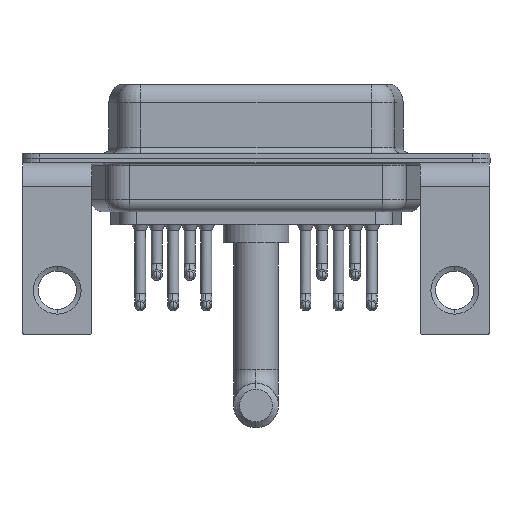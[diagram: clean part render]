
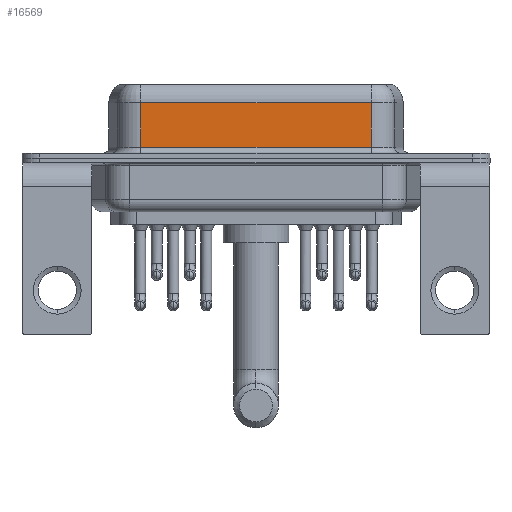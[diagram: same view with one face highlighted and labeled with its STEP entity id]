
A CAD part, front view. The second image highlights one B-rep face of the part: STEP entity #16569.
In plain terms, the highlighted planar face has unit normal (0, -1, 0).
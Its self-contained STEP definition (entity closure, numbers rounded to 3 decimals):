
#380 = PLANE ( 'NONE',  #9681 ) ;
#507 = DIRECTION ( 'NONE',  ( 1., 0., 0. ) ) ;
#1497 = ORIENTED_EDGE ( 'NONE', *, *, #11950, .T. ) ;
#1797 = ORIENTED_EDGE ( 'NONE', *, *, #18541, .T. ) ;
#2591 = LINE ( 'NONE', #11354, #2972 ) ;
#2831 = EDGE_LOOP ( 'NONE', ( #13888, #1497, #13884, #1797 ) ) ;
#2972 = VECTOR ( 'NONE', #3879, 1000. ) ;
#3325 = CARTESIAN_POINT ( 'NONE',  ( 7.013, -3.95, 4.65 ) ) ;
#3879 = DIRECTION ( 'NONE',  ( -1., 0., 0. ) ) ;
#4743 = CARTESIAN_POINT ( 'NONE',  ( 7.013, -3.95, 0.9 ) ) ;
#4881 = DIRECTION ( 'NONE',  ( 0., 0., 1. ) ) ;
#5713 = VECTOR ( 'NONE', #9147, 1000. ) ;
#6571 = VECTOR ( 'NONE', #507, 1000. ) ;
#6668 = EDGE_CURVE ( 'NONE', #12684, #18056, #15585, .T. ) ;
#7501 = EDGE_CURVE ( 'NONE', #17327, #13910, #16852, .T. ) ;
#9147 = DIRECTION ( 'NONE',  ( 0., 0., -1. ) ) ;
#9681 = AXIS2_PLACEMENT_3D ( 'NONE', #18183, #10700, #4881 ) ;
#10056 = CARTESIAN_POINT ( 'NONE',  ( 26.287, -3.95, 0.9 ) ) ;
#10700 = DIRECTION ( 'NONE',  ( 0., 1., 0. ) ) ;
#10924 = CARTESIAN_POINT ( 'NONE',  ( 26.287, -3.95, 0.9 ) ) ;
#11053 = DIRECTION ( 'NONE',  ( 0., 0., -1. ) ) ;
#11354 = CARTESIAN_POINT ( 'NONE',  ( 26.287, -3.95, 4.65 ) ) ;
#11950 = EDGE_CURVE ( 'NONE', #17327, #12684, #2591, .T. ) ;
#12113 = CARTESIAN_POINT ( 'NONE',  ( 26.287, -3.95, 6.4 ) ) ;
#12167 = FACE_OUTER_BOUND ( 'NONE', #2831, .T. ) ;
#12684 = VERTEX_POINT ( 'NONE', #3325 ) ;
#12723 = CARTESIAN_POINT ( 'NONE',  ( 7.013, -3.95, 6.4 ) ) ;
#13205 = VECTOR ( 'NONE', #11053, 1000. ) ;
#13884 = ORIENTED_EDGE ( 'NONE', *, *, #6668, .T. ) ;
#13888 = ORIENTED_EDGE ( 'NONE', *, *, #7501, .F. ) ;
#13910 = VERTEX_POINT ( 'NONE', #10056 ) ;
#15060 = CARTESIAN_POINT ( 'NONE',  ( 26.287, -3.95, 4.65 ) ) ;
#15585 = LINE ( 'NONE', #12723, #13205 ) ;
#16569 = ADVANCED_FACE ( 'NONE', ( #12167 ), #380, .F. ) ;
#16852 = LINE ( 'NONE', #12113, #5713 ) ;
#17327 = VERTEX_POINT ( 'NONE', #15060 ) ;
#18056 = VERTEX_POINT ( 'NONE', #4743 ) ;
#18183 = CARTESIAN_POINT ( 'NONE',  ( 26.287, -3.95, 6.4 ) ) ;
#18523 = LINE ( 'NONE', #10924, #6571 ) ;
#18541 = EDGE_CURVE ( 'NONE', #18056, #13910, #18523, .T. ) ;
